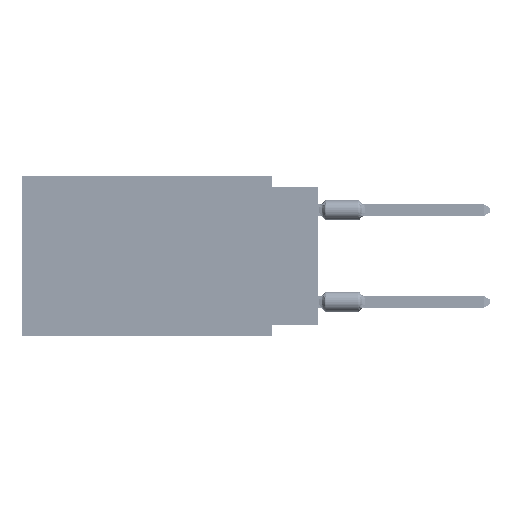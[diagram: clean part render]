
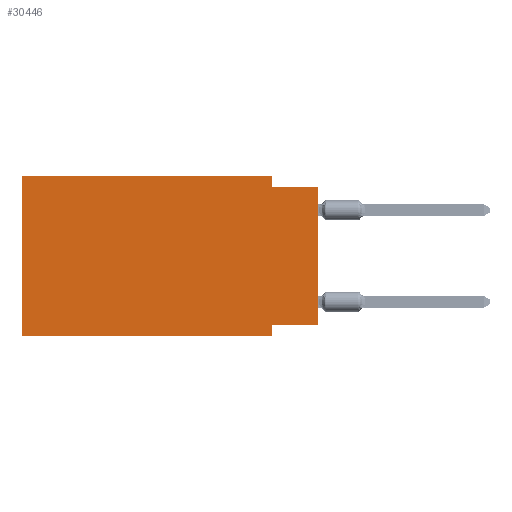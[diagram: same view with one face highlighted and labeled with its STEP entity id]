
A CAD part, left-side view. The second image highlights one B-rep face of the part: STEP entity #30446.
In plain terms, the highlighted planar face has unit normal (-1, 0, 0).
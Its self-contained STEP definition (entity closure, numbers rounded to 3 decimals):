
#606 = VERTEX_POINT ( 'NONE', #50889 ) ;
#923 = CARTESIAN_POINT ( 'NONE',  ( 0., 16.383, -8.89 ) ) ;
#2960 = DIRECTION ( 'NONE',  ( 0., -1., 0. ) ) ;
#5036 = AXIS2_PLACEMENT_3D ( 'NONE', #54194, #101037, #110748 ) ;
#5378 = EDGE_CURVE ( 'NONE', #7223, #98355, #14237, .T. ) ;
#7223 = VERTEX_POINT ( 'NONE', #923 ) ;
#7369 = LINE ( 'NONE', #49567, #51601 ) ;
#8827 = CARTESIAN_POINT ( 'NONE',  ( 0., 2.54, -8.89 ) ) ;
#9456 = VECTOR ( 'NONE', #82753, 1000. ) ;
#9742 = CARTESIAN_POINT ( 'NONE',  ( 0., 0., -8.255 ) ) ;
#11362 = EDGE_CURVE ( 'NONE', #31852, #94197, #45635, .T. ) ;
#12208 = VERTEX_POINT ( 'NONE', #24697 ) ;
#14237 = LINE ( 'NONE', #79320, #34742 ) ;
#15502 = ORIENTED_EDGE ( 'NONE', *, *, #11362, .F. ) ;
#17213 = VECTOR ( 'NONE', #2960, 1000. ) ;
#19352 = LINE ( 'NONE', #30880, #68988 ) ;
#24697 = CARTESIAN_POINT ( 'NONE',  ( 0., 2.54, 0. ) ) ;
#26900 = EDGE_LOOP ( 'NONE', ( #44804, #115395, #74867, #68473, #116559, #81868, #50651, #15502 ) ) ;
#30446 = ADVANCED_FACE ( 'NONE', ( #73684 ), #119256, .F. ) ;
#30880 = CARTESIAN_POINT ( 'NONE',  ( 0., 2.54, 0. ) ) ;
#31852 = VERTEX_POINT ( 'NONE', #66964 ) ;
#34742 = VECTOR ( 'NONE', #89629, 1000. ) ;
#40190 = EDGE_CURVE ( 'NONE', #82526, #606, #57696, .T. ) ;
#42827 = CARTESIAN_POINT ( 'NONE',  ( 0., 16.383, 0. ) ) ;
#43758 = CARTESIAN_POINT ( 'NONE',  ( 0., 0., 0. ) ) ;
#44804 = ORIENTED_EDGE ( 'NONE', *, *, #53304, .T. ) ;
#45115 = VECTOR ( 'NONE', #108824, 1000. ) ;
#45635 = LINE ( 'NONE', #9742, #9456 ) ;
#49567 = CARTESIAN_POINT ( 'NONE',  ( 0., 16.383, 0. ) ) ;
#50651 = ORIENTED_EDGE ( 'NONE', *, *, #114999, .F. ) ;
#50889 = CARTESIAN_POINT ( 'NONE',  ( 0., 0., -0.635 ) ) ;
#51601 = VECTOR ( 'NONE', #118041, 1000. ) ;
#53304 = EDGE_CURVE ( 'NONE', #31852, #606, #72937, .T. ) ;
#54194 = CARTESIAN_POINT ( 'NONE',  ( 0., 16.383, 0. ) ) ;
#57696 = LINE ( 'NONE', #68035, #17213 ) ;
#61408 = EDGE_CURVE ( 'NONE', #7223, #79223, #89048, .T. ) ;
#63252 = EDGE_CURVE ( 'NONE', #12208, #82526, #19352, .T. ) ;
#63851 = EDGE_CURVE ( 'NONE', #79223, #12208, #7369, .T. ) ;
#66964 = CARTESIAN_POINT ( 'NONE',  ( 0., 0., -8.255 ) ) ;
#67573 = DIRECTION ( 'NONE',  ( 0., 0., -1. ) ) ;
#68035 = CARTESIAN_POINT ( 'NONE',  ( 0., 0., -0.635 ) ) ;
#68473 = ORIENTED_EDGE ( 'NONE', *, *, #63851, .F. ) ;
#68786 = CARTESIAN_POINT ( 'NONE',  ( 0., 2.54, -8.89 ) ) ;
#68988 = VECTOR ( 'NONE', #75925, 1000. ) ;
#72937 = LINE ( 'NONE', #43758, #45115 ) ;
#73684 = FACE_OUTER_BOUND ( 'NONE', #26900, .T. ) ;
#74867 = ORIENTED_EDGE ( 'NONE', *, *, #63252, .F. ) ;
#75051 = CARTESIAN_POINT ( 'NONE',  ( 0., 2.54, -8.255 ) ) ;
#75925 = DIRECTION ( 'NONE',  ( 0., 0., -1. ) ) ;
#79223 = VERTEX_POINT ( 'NONE', #114772 ) ;
#79320 = CARTESIAN_POINT ( 'NONE',  ( 0., 16.383, -8.89 ) ) ;
#79810 = VECTOR ( 'NONE', #67573, 1000. ) ;
#81868 = ORIENTED_EDGE ( 'NONE', *, *, #5378, .T. ) ;
#82526 = VERTEX_POINT ( 'NONE', #86496 ) ;
#82753 = DIRECTION ( 'NONE',  ( 0., 1., 0. ) ) ;
#86496 = CARTESIAN_POINT ( 'NONE',  ( 0., 2.54, -0.635 ) ) ;
#89048 = LINE ( 'NONE', #42827, #93087 ) ;
#89629 = DIRECTION ( 'NONE',  ( 0., -1., 0. ) ) ;
#90843 = DIRECTION ( 'NONE',  ( 0., 0., 1. ) ) ;
#93087 = VECTOR ( 'NONE', #90843, 1000. ) ;
#94197 = VERTEX_POINT ( 'NONE', #75051 ) ;
#98355 = VERTEX_POINT ( 'NONE', #8827 ) ;
#101037 = DIRECTION ( 'NONE',  ( 1., 0., 0. ) ) ;
#108824 = DIRECTION ( 'NONE',  ( 0., 0., 1. ) ) ;
#110748 = DIRECTION ( 'NONE',  ( 0., 0., -1. ) ) ;
#114772 = CARTESIAN_POINT ( 'NONE',  ( 0., 16.383, 0. ) ) ;
#114999 = EDGE_CURVE ( 'NONE', #94197, #98355, #115559, .T. ) ;
#115395 = ORIENTED_EDGE ( 'NONE', *, *, #40190, .F. ) ;
#115559 = LINE ( 'NONE', #68786, #79810 ) ;
#116559 = ORIENTED_EDGE ( 'NONE', *, *, #61408, .F. ) ;
#118041 = DIRECTION ( 'NONE',  ( 0., -1., 0. ) ) ;
#119256 = PLANE ( 'NONE',  #5036 ) ;
